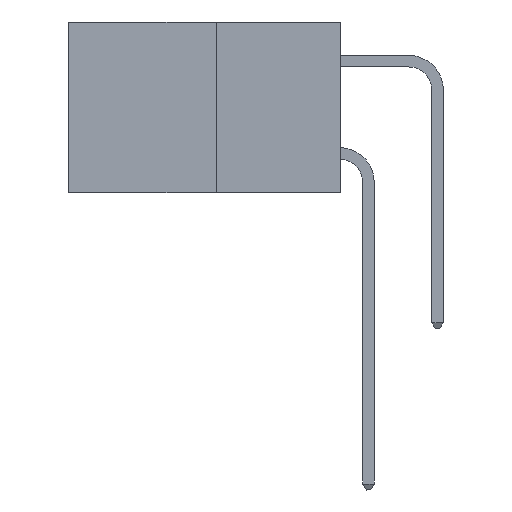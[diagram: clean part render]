
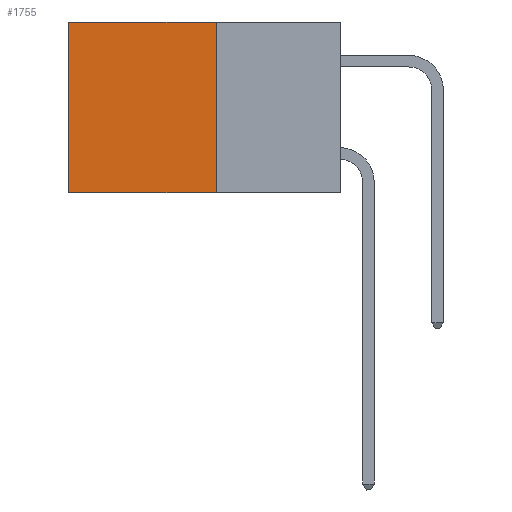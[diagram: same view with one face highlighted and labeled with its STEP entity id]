
A CAD part, left-side view. The second image highlights one B-rep face of the part: STEP entity #1755.
In plain terms, the highlighted planar face has unit normal (-1, 0, 0).
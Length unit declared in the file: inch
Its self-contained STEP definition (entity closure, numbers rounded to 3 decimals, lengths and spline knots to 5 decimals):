
#704 = CARTESIAN_POINT ( 'NONE',  ( 0.277, 0.59, 0. ) ) ;
#1011 = VECTOR ( 'NONE', #6800, 39.37008 ) ;
#1755 = ADVANCED_FACE ( 'NONE', ( #9008 ), #16233, .F. ) ;
#1940 = EDGE_LOOP ( 'NONE', ( #4429, #17138, #2677, #14151 ) ) ;
#2206 = VECTOR ( 'NONE', #15965, 39.37008 ) ;
#2677 = ORIENTED_EDGE ( 'NONE', *, *, #6600, .F. ) ;
#2873 = VECTOR ( 'NONE', #4966, 39.37008 ) ;
#3337 = CARTESIAN_POINT ( 'NONE',  ( 0.277, 0.27, -0.37 ) ) ;
#4046 = AXIS2_PLACEMENT_3D ( 'NONE', #17676, #19528, #18669 ) ;
#4429 = ORIENTED_EDGE ( 'NONE', *, *, #11157, .T. ) ;
#4966 = DIRECTION ( 'NONE',  ( 0., 1., 0. ) ) ;
#5047 = CARTESIAN_POINT ( 'NONE',  ( 0.277, 0.59, -0.37 ) ) ;
#5127 = CARTESIAN_POINT ( 'NONE',  ( 0.277, 0.27, 0. ) ) ;
#5924 = LINE ( 'NONE', #9961, #2206 ) ;
#6318 = VERTEX_POINT ( 'NONE', #5127 ) ;
#6600 = EDGE_CURVE ( 'NONE', #6318, #12422, #8313, .T. ) ;
#6664 = DIRECTION ( 'NONE',  ( 0., 0., -1. ) ) ;
#6800 = DIRECTION ( 'NONE',  ( 0., 0., -1. ) ) ;
#6948 = CARTESIAN_POINT ( 'NONE',  ( 0.277, 0.27, -0.37 ) ) ;
#7223 = LINE ( 'NONE', #5047, #18630 ) ;
#7877 = EDGE_CURVE ( 'NONE', #6318, #11979, #5924, .T. ) ;
#8313 = LINE ( 'NONE', #6948, #1011 ) ;
#9008 = FACE_OUTER_BOUND ( 'NONE', #1940, .T. ) ;
#9536 = CARTESIAN_POINT ( 'NONE',  ( 0.277, 0.59, -0.37 ) ) ;
#9961 = CARTESIAN_POINT ( 'NONE',  ( 0.277, 0.27, 0. ) ) ;
#11157 = EDGE_CURVE ( 'NONE', #11979, #18802, #7223, .T. ) ;
#11979 = VERTEX_POINT ( 'NONE', #704 ) ;
#12422 = VERTEX_POINT ( 'NONE', #3337 ) ;
#14114 = CARTESIAN_POINT ( 'NONE',  ( 0.277, 0.27, -0.37 ) ) ;
#14151 = ORIENTED_EDGE ( 'NONE', *, *, #7877, .T. ) ;
#15965 = DIRECTION ( 'NONE',  ( 0., 1., 0. ) ) ;
#16233 = PLANE ( 'NONE',  #4046 ) ;
#16498 = EDGE_CURVE ( 'NONE', #12422, #18802, #18953, .T. ) ;
#17138 = ORIENTED_EDGE ( 'NONE', *, *, #16498, .F. ) ;
#17676 = CARTESIAN_POINT ( 'NONE',  ( 0.277, 0.27, -0.37 ) ) ;
#18630 = VECTOR ( 'NONE', #6664, 39.37008 ) ;
#18669 = DIRECTION ( 'NONE',  ( 0., 0., -1. ) ) ;
#18802 = VERTEX_POINT ( 'NONE', #9536 ) ;
#18953 = LINE ( 'NONE', #14114, #2873 ) ;
#19528 = DIRECTION ( 'NONE',  ( 1., 0., 0. ) ) ;
